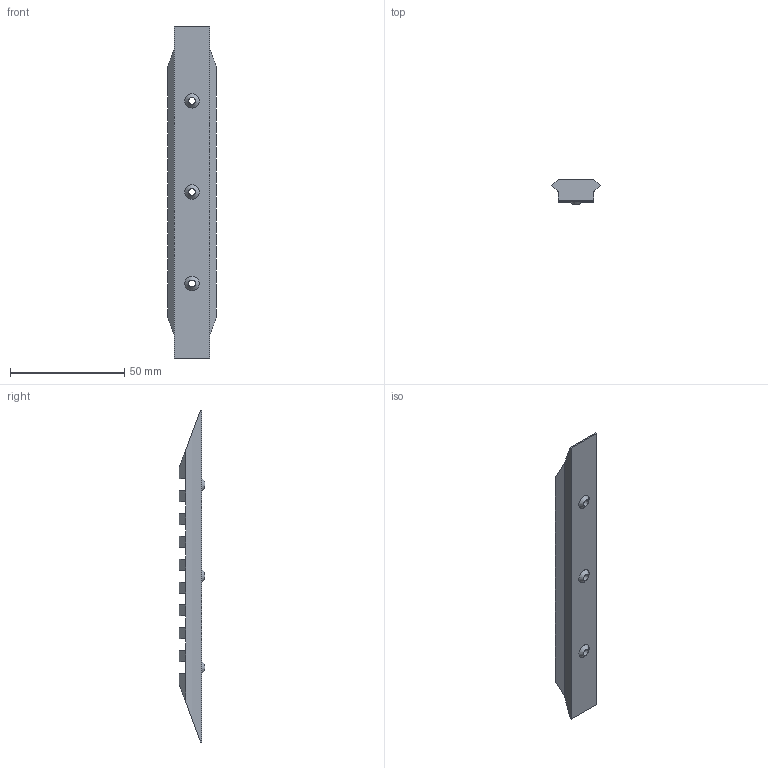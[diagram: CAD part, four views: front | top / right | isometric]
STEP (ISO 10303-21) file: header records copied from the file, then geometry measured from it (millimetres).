
FILE_DESCRIPTION(/* description */ (''),/* implementation_level */ '2;1');
FILE_NAME(/* name */ 'Ivan''Top Rail.stp',/* time_stamp */ '2020-06-26T16:22:39-05:00',/* author */ ('johne'),/* organization */ (''),/* preprocessor_version */ 'ST-DEVELOPER v18',/* originating_system */ 'Autodesk Inventor 2020',/* authorisation */ '');
FILE_SCHEMA (('AUTOMOTIVE_DESIGN { 1 0 10303 214 3 1 1 }'));
Length unit declared in the file: inch
Products named in the file (1): Top Rail
Bounding box: 21.2 x 11.21 x 145.4 mm (x, y, z)
Volume: 17834 mm3; surface area: 8793.5 mm2
Topology: 1 solids, 1 shells, 93 faces, 234 edges, 146 vertices
Faces by surface type: plane 81, cylinder 9, cone 3
Full cylindrical faces by diameter (mm): 3 x3, 6.35 x6
Entity records: 2785 total; most frequent: CARTESIAN_POINT 474, ORIENTED_EDGE 468, DIRECTION 464, EDGE_CURVE 234, LINE 192, VECTOR 192, VERTEX_POINT 146, AXIS2_PLACEMENT_3D 136
